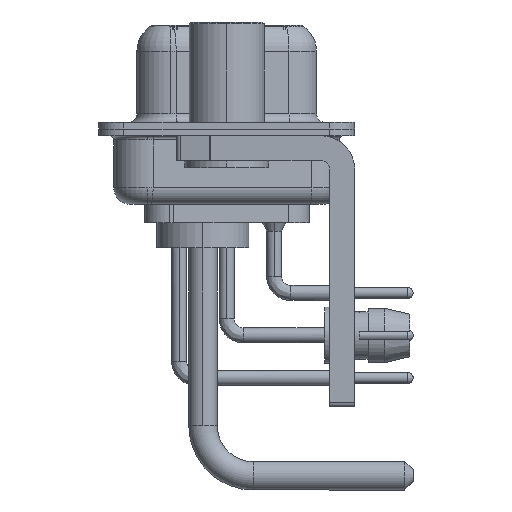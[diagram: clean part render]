
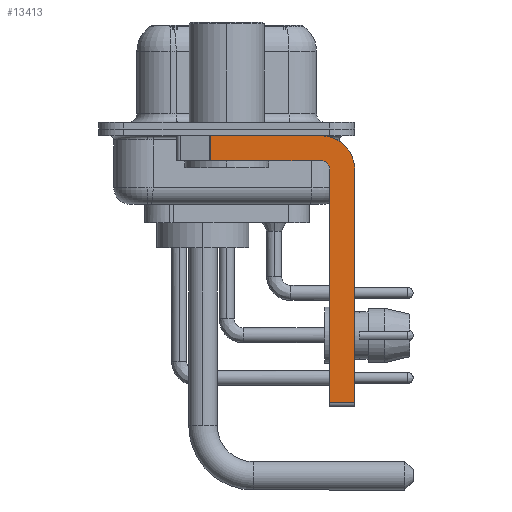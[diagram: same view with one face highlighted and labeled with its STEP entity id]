
A CAD part, left-side view. The second image highlights one B-rep face of the part: STEP entity #13413.
In plain terms, the highlighted planar face has unit normal (-1, 0, 0).
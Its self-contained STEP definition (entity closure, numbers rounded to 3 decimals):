
#2503 = VERTEX_POINT ( 'NONE', #19286 ) ;
#2844 = CARTESIAN_POINT ( 'NONE',  ( -2.9, -5.65, -2.4 ) ) ;
#3504 = ORIENTED_EDGE ( 'NONE', *, *, #29139, .T. ) ;
#3651 = CARTESIAN_POINT ( 'NONE',  ( -2.9, -6.15, -16.35 ) ) ;
#3794 = ORIENTED_EDGE ( 'NONE', *, *, #28921, .F. ) ;
#4414 = DIRECTION ( 'NONE',  ( 1., 0., 0. ) ) ;
#4815 = CIRCLE ( 'NONE', #18729, 0.5 ) ;
#4923 = DIRECTION ( 'NONE',  ( 0., -1., 0. ) ) ;
#4929 = VERTEX_POINT ( 'NONE', #28819 ) ;
#5028 = EDGE_CURVE ( 'NONE', #28703, #6917, #14231, .T. ) ;
#5640 = CARTESIAN_POINT ( 'NONE',  ( -2.9, -6.15, -16.6 ) ) ;
#5984 = VERTEX_POINT ( 'NONE', #28730 ) ;
#6482 = EDGE_CURVE ( 'NONE', #17446, #19887, #36412, .T. ) ;
#6917 = VERTEX_POINT ( 'NONE', #23828 ) ;
#9101 = EDGE_CURVE ( 'NONE', #2503, #20945, #4815, .T. ) ;
#9207 = ORIENTED_EDGE ( 'NONE', *, *, #9101, .F. ) ;
#10600 = EDGE_LOOP ( 'NONE', ( #27925, #3504, #22009, #9207, #20270, #18351, #15183, #3794 ) ) ;
#11216 = EDGE_CURVE ( 'NONE', #20945, #5984, #35421, .T. ) ;
#11735 = PLANE ( 'NONE',  #31631 ) ;
#13413 = ADVANCED_FACE ( 'NONE', ( #17072 ), #11735, .F. ) ;
#14169 = LINE ( 'NONE', #5640, #24037 ) ;
#14231 = LINE ( 'NONE', #25783, #22185 ) ;
#14250 = DIRECTION ( 'NONE',  ( 0., 0., -1. ) ) ;
#14589 = DIRECTION ( 'NONE',  ( 1., 0., 0. ) ) ;
#15183 = ORIENTED_EDGE ( 'NONE', *, *, #24025, .F. ) ;
#16601 = EDGE_CURVE ( 'NONE', #28703, #2503, #14169, .T. ) ;
#17072 = FACE_OUTER_BOUND ( 'NONE', #10600, .T. ) ;
#17446 = VERTEX_POINT ( 'NONE', #34324 ) ;
#18351 = ORIENTED_EDGE ( 'NONE', *, *, #5028, .T. ) ;
#18729 = AXIS2_PLACEMENT_3D ( 'NONE', #25780, #37370, #34715 ) ;
#19286 = CARTESIAN_POINT ( 'NONE',  ( -2.9, -6.15, -2.4 ) ) ;
#19887 = VERTEX_POINT ( 'NONE', #35735 ) ;
#20270 = ORIENTED_EDGE ( 'NONE', *, *, #16601, .F. ) ;
#20945 = VERTEX_POINT ( 'NONE', #34784 ) ;
#21170 = CARTESIAN_POINT ( 'NONE',  ( -2.9, -5.65, -1.9 ) ) ;
#22009 = ORIENTED_EDGE ( 'NONE', *, *, #11216, .F. ) ;
#22017 = DIRECTION ( 'NONE',  ( 0., 0., -1. ) ) ;
#22185 = VECTOR ( 'NONE', #23866, 1000. ) ;
#23828 = CARTESIAN_POINT ( 'NONE',  ( -2.9, -7.65, -16.35 ) ) ;
#23866 = DIRECTION ( 'NONE',  ( 0., -1., 0. ) ) ;
#24025 = EDGE_CURVE ( 'NONE', #4929, #6917, #36448, .T. ) ;
#24037 = VECTOR ( 'NONE', #28753, 1000. ) ;
#24197 = DIRECTION ( 'NONE',  ( 0., 1., 0. ) ) ;
#25780 = CARTESIAN_POINT ( 'NONE',  ( -2.9, -5.65, -2.4 ) ) ;
#25783 = CARTESIAN_POINT ( 'NONE',  ( -2.9, -5.65, -16.35 ) ) ;
#26174 = VECTOR ( 'NONE', #22017, 1000. ) ;
#27279 = CARTESIAN_POINT ( 'NONE',  ( -2.9, 3., -0.4 ) ) ;
#27313 = CARTESIAN_POINT ( 'NONE',  ( -2.9, -7.65, -2.4 ) ) ;
#27925 = ORIENTED_EDGE ( 'NONE', *, *, #6482, .F. ) ;
#28703 = VERTEX_POINT ( 'NONE', #3651 ) ;
#28730 = CARTESIAN_POINT ( 'NONE',  ( -2.9, 0.978, -1.9 ) ) ;
#28753 = DIRECTION ( 'NONE',  ( 0., 0., 1. ) ) ;
#28819 = CARTESIAN_POINT ( 'NONE',  ( -2.9, -7.65, -2.4 ) ) ;
#28921 = EDGE_CURVE ( 'NONE', #19887, #4929, #33993, .T. ) ;
#29139 = EDGE_CURVE ( 'NONE', #17446, #5984, #29405, .T. ) ;
#29405 = LINE ( 'NONE', #31703, #35823 ) ;
#29740 = AXIS2_PLACEMENT_3D ( 'NONE', #30383, #4414, #36275 ) ;
#30383 = CARTESIAN_POINT ( 'NONE',  ( -2.9, -5.65, -2.4 ) ) ;
#31631 = AXIS2_PLACEMENT_3D ( 'NONE', #2844, #14589, #37014 ) ;
#31703 = CARTESIAN_POINT ( 'NONE',  ( -2.9, 0.978, -1.9 ) ) ;
#33993 = CIRCLE ( 'NONE', #29740, 2. ) ;
#34324 = CARTESIAN_POINT ( 'NONE',  ( -2.9, 0.978, -0.4 ) ) ;
#34611 = VECTOR ( 'NONE', #24197, 1000. ) ;
#34715 = DIRECTION ( 'NONE',  ( 0., 0., 1. ) ) ;
#34784 = CARTESIAN_POINT ( 'NONE',  ( -2.9, -5.65, -1.9 ) ) ;
#35421 = LINE ( 'NONE', #21170, #34611 ) ;
#35623 = VECTOR ( 'NONE', #4923, 1000. ) ;
#35735 = CARTESIAN_POINT ( 'NONE',  ( -2.9, -5.65, -0.4 ) ) ;
#35823 = VECTOR ( 'NONE', #14250, 1000. ) ;
#36275 = DIRECTION ( 'NONE',  ( 0., 0., -1. ) ) ;
#36412 = LINE ( 'NONE', #27279, #35623 ) ;
#36448 = LINE ( 'NONE', #27313, #26174 ) ;
#37014 = DIRECTION ( 'NONE',  ( 0., 0., -1. ) ) ;
#37370 = DIRECTION ( 'NONE',  ( -1., 0., 0. ) ) ;
